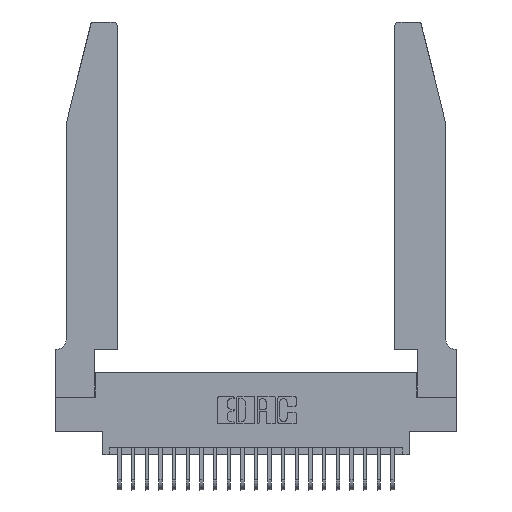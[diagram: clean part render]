
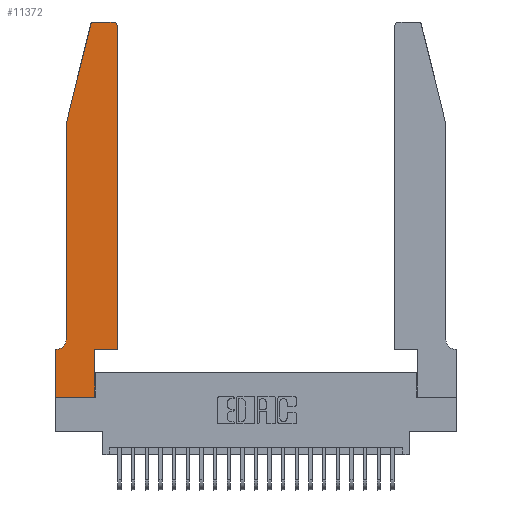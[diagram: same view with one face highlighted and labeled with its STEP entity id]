
A CAD part, top view. The second image highlights one B-rep face of the part: STEP entity #11372.
In plain terms, the highlighted planar face has unit normal (0, 0, 1).
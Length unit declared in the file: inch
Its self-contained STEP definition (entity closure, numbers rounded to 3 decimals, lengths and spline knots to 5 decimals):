
#408 = CARTESIAN_POINT ( 'NONE',  ( 0.25487, 2.72718, 0.37 ) ) ;
#479 = VECTOR ( 'NONE', #1785, 39.37008 ) ;
#788 = VECTOR ( 'NONE', #16048, 39.37008 ) ;
#846 = FACE_OUTER_BOUND ( 'NONE', #12000, .T. ) ;
#1208 = DIRECTION ( 'NONE',  ( 1., 0., 0. ) ) ;
#1306 = CARTESIAN_POINT ( 'NONE',  ( 0.0755, 2., 0.37 ) ) ;
#1670 = EDGE_CURVE ( 'NONE', #15970, #6000, #4570, .T. ) ;
#1761 = CARTESIAN_POINT ( 'NONE',  ( 0.0755, 2., 0.37 ) ) ;
#1785 = DIRECTION ( 'NONE',  ( -1., 0., 0. ) ) ;
#2044 = DIRECTION ( 'NONE',  ( 1., 0., 0. ) ) ;
#2079 = DIRECTION ( 'NONE',  ( 0., 0., 1. ) ) ;
#2147 = EDGE_CURVE ( 'NONE', #18097, #2854, #25654, .T. ) ;
#2224 = CARTESIAN_POINT ( 'NONE',  ( 0.284, 2.72, 0.37 ) ) ;
#2286 = VECTOR ( 'NONE', #3551, 39.37008 ) ;
#2854 = VERTEX_POINT ( 'NONE', #408 ) ;
#3358 = VECTOR ( 'NONE', #3384, 39.37008 ) ;
#3384 = DIRECTION ( 'NONE',  ( -0.239, -0.971, 0. ) ) ;
#3547 = CARTESIAN_POINT ( 'NONE',  ( 0.4505, 0.35, 0.37 ) ) ;
#3551 = DIRECTION ( 'NONE',  ( -1., 0., 0. ) ) ;
#4362 = LINE ( 'NONE', #3547, #24872 ) ;
#4398 = ORIENTED_EDGE ( 'NONE', *, *, #18242, .T. ) ;
#4477 = CARTESIAN_POINT ( 'NONE',  ( 0.0755, 2., 0.37 ) ) ;
#4570 = LINE ( 'NONE', #23630, #14791 ) ;
#5559 = CARTESIAN_POINT ( 'NONE',  ( 0.4505, 2.72, 0.37 ) ) ;
#6000 = VERTEX_POINT ( 'NONE', #18785 ) ;
#6084 = ORIENTED_EDGE ( 'NONE', *, *, #12138, .T. ) ;
#6693 = CARTESIAN_POINT ( 'NONE',  ( 0.4205, 2.72, 0.37 ) ) ;
#7088 = DIRECTION ( 'NONE',  ( 0., -1., 0. ) ) ;
#7104 = EDGE_CURVE ( 'NONE', #14709, #13437, #11760, .T. ) ;
#7109 = LINE ( 'NONE', #17712, #2286 ) ;
#7843 = DIRECTION ( 'NONE',  ( 0., 0., -1. ) ) ;
#8268 = ORIENTED_EDGE ( 'NONE', *, *, #7104, .T. ) ;
#8801 = DIRECTION ( 'NONE',  ( 1., 0., 0. ) ) ;
#9335 = CARTESIAN_POINT ( 'NONE',  ( 0.0055, 0.35, 0.37 ) ) ;
#9610 = EDGE_CURVE ( 'NONE', #6000, #24339, #17468, .T. ) ;
#9779 = DIRECTION ( 'NONE',  ( 0., 0., 1. ) ) ;
#10337 = CARTESIAN_POINT ( 'NONE',  ( 0.284, 2.75, 0.37 ) ) ;
#10522 = CARTESIAN_POINT ( 'NONE',  ( 0.4205, 2.75, 0.37 ) ) ;
#10957 = ORIENTED_EDGE ( 'NONE', *, *, #11107, .T. ) ;
#11107 = EDGE_CURVE ( 'NONE', #23429, #14658, #21925, .T. ) ;
#11372 = ADVANCED_FACE ( 'NONE', ( #846 ), #13745, .T. ) ;
#11651 = CARTESIAN_POINT ( 'NONE',  ( 0.0755, 0.42, 0.37 ) ) ;
#11760 = LINE ( 'NONE', #1761, #788 ) ;
#11845 = DIRECTION ( 'NONE',  ( 0., 1., 0. ) ) ;
#12000 = EDGE_LOOP ( 'NONE', ( #16170, #16900, #13207, #8268, #18882, #6084, #15359, #4398, #13752, #20743, #15030, #10957 ) ) ;
#12138 = EDGE_CURVE ( 'NONE', #24565, #14947, #16753, .T. ) ;
#12227 = VECTOR ( 'NONE', #1208, 39.37008 ) ;
#12358 = CARTESIAN_POINT ( 'NONE',  ( 0.2865, 0., 0.37 ) ) ;
#12708 = EDGE_CURVE ( 'NONE', #2854, #14709, #14223, .T. ) ;
#12926 = CARTESIAN_POINT ( 'NONE',  ( 0., 0., 0.37 ) ) ;
#13207 = ORIENTED_EDGE ( 'NONE', *, *, #12708, .T. ) ;
#13437 = VERTEX_POINT ( 'NONE', #11651 ) ;
#13524 = CARTESIAN_POINT ( 'NONE',  ( 0.4505, 0.35, 0.37 ) ) ;
#13745 = PLANE ( 'NONE',  #14994 ) ;
#13752 = ORIENTED_EDGE ( 'NONE', *, *, #1670, .T. ) ;
#13798 = VERTEX_POINT ( 'NONE', #20644 ) ;
#14027 = CIRCLE ( 'NONE', #16280, 0.07 ) ;
#14045 = CARTESIAN_POINT ( 'NONE',  ( 0.0755, 0.35, 0.37 ) ) ;
#14223 = LINE ( 'NONE', #1306, #3358 ) ;
#14535 = LINE ( 'NONE', #17164, #19733 ) ;
#14658 = VERTEX_POINT ( 'NONE', #10522 ) ;
#14709 = VERTEX_POINT ( 'NONE', #4477 ) ;
#14791 = VECTOR ( 'NONE', #15289, 39.37008 ) ;
#14947 = VERTEX_POINT ( 'NONE', #21112 ) ;
#14994 = AXIS2_PLACEMENT_3D ( 'NONE', #21587, #9779, #23495 ) ;
#15030 = ORIENTED_EDGE ( 'NONE', *, *, #18579, .T. ) ;
#15289 = DIRECTION ( 'NONE',  ( 0., 1., 0. ) ) ;
#15359 = ORIENTED_EDGE ( 'NONE', *, *, #19492, .T. ) ;
#15970 = VERTEX_POINT ( 'NONE', #12358 ) ;
#16048 = DIRECTION ( 'NONE',  ( 0., -1., 0. ) ) ;
#16170 = ORIENTED_EDGE ( 'NONE', *, *, #25791, .T. ) ;
#16280 = AXIS2_PLACEMENT_3D ( 'NONE', #19802, #7843, #21733 ) ;
#16753 = LINE ( 'NONE', #14045, #479 ) ;
#16807 = AXIS2_PLACEMENT_3D ( 'NONE', #6693, #20682, #8801 ) ;
#16900 = ORIENTED_EDGE ( 'NONE', *, *, #2147, .T. ) ;
#17164 = CARTESIAN_POINT ( 'NONE',  ( 0., 0., 0.37 ) ) ;
#17277 = EDGE_CURVE ( 'NONE', #13437, #24565, #14027, .T. ) ;
#17468 = LINE ( 'NONE', #13524, #12227 ) ;
#17712 = CARTESIAN_POINT ( 'NONE',  ( 0.2605, 2.75, 0.37 ) ) ;
#17985 = VECTOR ( 'NONE', #24527, 39.37008 ) ;
#18097 = VERTEX_POINT ( 'NONE', #10337 ) ;
#18242 = EDGE_CURVE ( 'NONE', #13798, #15970, #22514, .T. ) ;
#18579 = EDGE_CURVE ( 'NONE', #24339, #23429, #4362, .T. ) ;
#18785 = CARTESIAN_POINT ( 'NONE',  ( 0.2865, 0.35, 0.37 ) ) ;
#18882 = ORIENTED_EDGE ( 'NONE', *, *, #17277, .T. ) ;
#19492 = EDGE_CURVE ( 'NONE', #14947, #13798, #14535, .T. ) ;
#19733 = VECTOR ( 'NONE', #7088, 39.37008 ) ;
#19802 = CARTESIAN_POINT ( 'NONE',  ( 0.0055, 0.42, 0.37 ) ) ;
#20257 = AXIS2_PLACEMENT_3D ( 'NONE', #2224, #2079, #2044 ) ;
#20644 = CARTESIAN_POINT ( 'NONE',  ( 0., 0., 0.37 ) ) ;
#20682 = DIRECTION ( 'NONE',  ( 0., 0., 1. ) ) ;
#20743 = ORIENTED_EDGE ( 'NONE', *, *, #9610, .T. ) ;
#21112 = CARTESIAN_POINT ( 'NONE',  ( 0., 0.35, 0.37 ) ) ;
#21587 = CARTESIAN_POINT ( 'NONE',  ( 0., 0.35, 0.37 ) ) ;
#21733 = DIRECTION ( 'NONE',  ( -1., 0., 0. ) ) ;
#21925 = CIRCLE ( 'NONE', #16807, 0.03 ) ;
#22357 = CARTESIAN_POINT ( 'NONE',  ( 0.4505, 0.35, 0.37 ) ) ;
#22514 = LINE ( 'NONE', #12926, #17985 ) ;
#23429 = VERTEX_POINT ( 'NONE', #5559 ) ;
#23495 = DIRECTION ( 'NONE',  ( 1., 0., 0. ) ) ;
#23630 = CARTESIAN_POINT ( 'NONE',  ( 0.2865, 0.35, 0.37 ) ) ;
#24339 = VERTEX_POINT ( 'NONE', #22357 ) ;
#24527 = DIRECTION ( 'NONE',  ( 1., 0., 0. ) ) ;
#24565 = VERTEX_POINT ( 'NONE', #9335 ) ;
#24872 = VECTOR ( 'NONE', #11845, 39.37008 ) ;
#25654 = CIRCLE ( 'NONE', #20257, 0.03 ) ;
#25791 = EDGE_CURVE ( 'NONE', #14658, #18097, #7109, .T. ) ;
